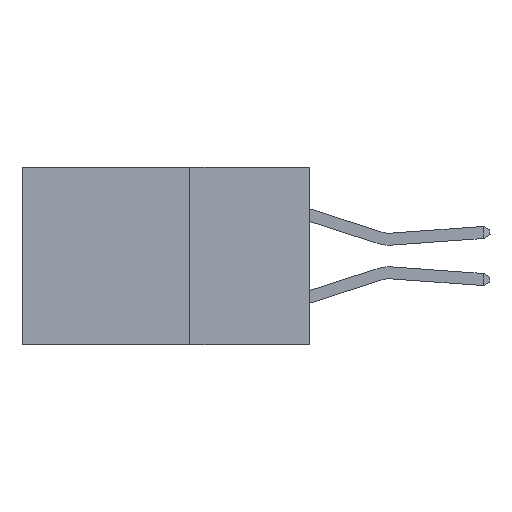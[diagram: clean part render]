
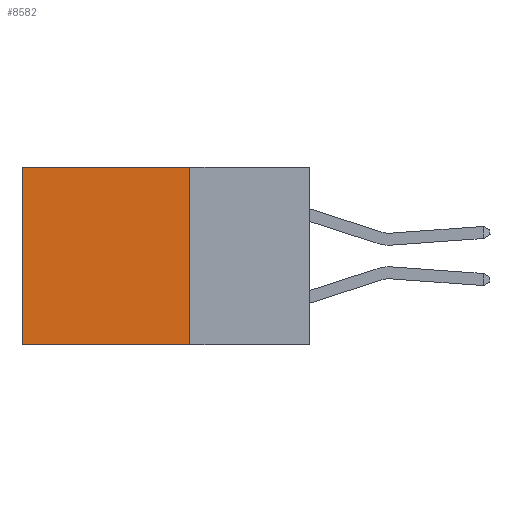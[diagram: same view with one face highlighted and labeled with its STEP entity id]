
A CAD part, left-side view. The second image highlights one B-rep face of the part: STEP entity #8582.
In plain terms, the highlighted planar face has unit normal (-1, 0, 0).
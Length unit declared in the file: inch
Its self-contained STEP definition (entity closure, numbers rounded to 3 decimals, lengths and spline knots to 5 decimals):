
#139 = CARTESIAN_POINT ( 'NONE',  ( 0.2615, 0.25, 0. ) ) ;
#983 = EDGE_CURVE ( 'NONE', #4545, #8295, #5975, .T. ) ;
#1363 = DIRECTION ( 'NONE',  ( 0., 1., 0. ) ) ;
#2212 = ORIENTED_EDGE ( 'NONE', *, *, #983, .F. ) ;
#2406 = LINE ( 'NONE', #8208, #2821 ) ;
#2821 = VECTOR ( 'NONE', #1363, 39.37008 ) ;
#3218 = CARTESIAN_POINT ( 'NONE',  ( 0.2615, 0.25, -0.37 ) ) ;
#3415 = EDGE_CURVE ( 'NONE', #4597, #7159, #7343, .T. ) ;
#3480 = DIRECTION ( 'NONE',  ( 0., 1., 0. ) ) ;
#3883 = CARTESIAN_POINT ( 'NONE',  ( 0.2615, 0.6, -0.37 ) ) ;
#3892 = DIRECTION ( 'NONE',  ( 0., 0., -1. ) ) ;
#4031 = ORIENTED_EDGE ( 'NONE', *, *, #7071, .T. ) ;
#4328 = CARTESIAN_POINT ( 'NONE',  ( 0.2615, 0.25, 0. ) ) ;
#4434 = CARTESIAN_POINT ( 'NONE',  ( 0.2615, 0.6, 0. ) ) ;
#4545 = VERTEX_POINT ( 'NONE', #4328 ) ;
#4597 = VERTEX_POINT ( 'NONE', #4434 ) ;
#4779 = CARTESIAN_POINT ( 'NONE',  ( 0.2615, 0.25, -0.37 ) ) ;
#4921 = FACE_OUTER_BOUND ( 'NONE', #7682, .T. ) ;
#5975 = LINE ( 'NONE', #7624, #8271 ) ;
#6529 = PLANE ( 'NONE',  #7345 ) ;
#6601 = ORIENTED_EDGE ( 'NONE', *, *, #8703, .F. ) ;
#7071 = EDGE_CURVE ( 'NONE', #4545, #4597, #10293, .T. ) ;
#7096 = VECTOR ( 'NONE', #3480, 39.37008 ) ;
#7159 = VERTEX_POINT ( 'NONE', #7289 ) ;
#7289 = CARTESIAN_POINT ( 'NONE',  ( 0.2615, 0.6, -0.37 ) ) ;
#7343 = LINE ( 'NONE', #3883, #9015 ) ;
#7345 = AXIS2_PLACEMENT_3D ( 'NONE', #3218, #8056, #3892 ) ;
#7624 = CARTESIAN_POINT ( 'NONE',  ( 0.2615, 0.25, -0.37 ) ) ;
#7682 = EDGE_LOOP ( 'NONE', ( #8844, #6601, #2212, #4031 ) ) ;
#8056 = DIRECTION ( 'NONE',  ( 1., 0., 0. ) ) ;
#8208 = CARTESIAN_POINT ( 'NONE',  ( 0.2615, 0.25, -0.37 ) ) ;
#8271 = VECTOR ( 'NONE', #9315, 39.37008 ) ;
#8295 = VERTEX_POINT ( 'NONE', #4779 ) ;
#8582 = ADVANCED_FACE ( 'NONE', ( #4921 ), #6529, .F. ) ;
#8703 = EDGE_CURVE ( 'NONE', #8295, #7159, #2406, .T. ) ;
#8844 = ORIENTED_EDGE ( 'NONE', *, *, #3415, .T. ) ;
#9015 = VECTOR ( 'NONE', #10679, 39.37008 ) ;
#9315 = DIRECTION ( 'NONE',  ( 0., 0., -1. ) ) ;
#10293 = LINE ( 'NONE', #139, #7096 ) ;
#10679 = DIRECTION ( 'NONE',  ( 0., 0., -1. ) ) ;
